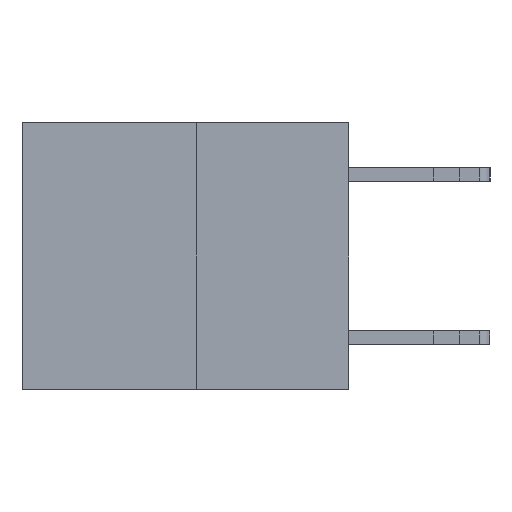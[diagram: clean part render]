
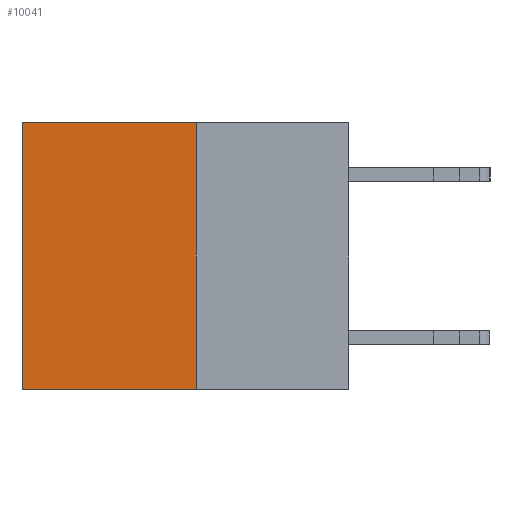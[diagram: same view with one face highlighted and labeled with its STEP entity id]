
A CAD part, left-side view. The second image highlights one B-rep face of the part: STEP entity #10041.
In plain terms, the highlighted planar face has unit normal (-1, 0, 0).
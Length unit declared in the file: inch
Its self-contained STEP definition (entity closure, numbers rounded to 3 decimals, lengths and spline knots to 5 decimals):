
#170 = PLANE ( 'NONE',  #9538 ) ;
#248 = CARTESIAN_POINT ( 'NONE',  ( 0.3165, 0.28, -0.49 ) ) ;
#251 = DIRECTION ( 'NONE',  ( 0., 1., 0. ) ) ;
#1342 = ORIENTED_EDGE ( 'NONE', *, *, #8100, .F. ) ;
#1426 = EDGE_CURVE ( 'NONE', #12046, #2848, #7348, .T. ) ;
#1873 = EDGE_LOOP ( 'NONE', ( #5489, #9481, #1342, #3437 ) ) ;
#2848 = VERTEX_POINT ( 'NONE', #3952 ) ;
#2997 = EDGE_CURVE ( 'NONE', #3380, #7365, #10360, .T. ) ;
#3380 = VERTEX_POINT ( 'NONE', #11520 ) ;
#3437 = ORIENTED_EDGE ( 'NONE', *, *, #1426, .T. ) ;
#3952 = CARTESIAN_POINT ( 'NONE',  ( 0.3165, 0.6, 0. ) ) ;
#4978 = LINE ( 'NONE', #10713, #12316 ) ;
#5038 = VECTOR ( 'NONE', #5863, 39.37008 ) ;
#5358 = CARTESIAN_POINT ( 'NONE',  ( 0.3165, 0.28, 0. ) ) ;
#5463 = VECTOR ( 'NONE', #251, 39.37008 ) ;
#5489 = ORIENTED_EDGE ( 'NONE', *, *, #10489, .T. ) ;
#5657 = DIRECTION ( 'NONE',  ( 0., 0., -1. ) ) ;
#5863 = DIRECTION ( 'NONE',  ( 0., 1., 0. ) ) ;
#6098 = CARTESIAN_POINT ( 'NONE',  ( 0.3165, 0.28, -0.49 ) ) ;
#6902 = DIRECTION ( 'NONE',  ( 1., 0., 0. ) ) ;
#7070 = VECTOR ( 'NONE', #5657, 39.37008 ) ;
#7348 = LINE ( 'NONE', #10740, #5038 ) ;
#7365 = VERTEX_POINT ( 'NONE', #9701 ) ;
#7507 = CARTESIAN_POINT ( 'NONE',  ( 0.3165, 0.28, -0.49 ) ) ;
#7882 = DIRECTION ( 'NONE',  ( 0., 0., -1. ) ) ;
#7975 = LINE ( 'NONE', #7507, #7070 ) ;
#8100 = EDGE_CURVE ( 'NONE', #12046, #3380, #7975, .T. ) ;
#9481 = ORIENTED_EDGE ( 'NONE', *, *, #2997, .F. ) ;
#9538 = AXIS2_PLACEMENT_3D ( 'NONE', #248, #6902, #7882 ) ;
#9701 = CARTESIAN_POINT ( 'NONE',  ( 0.3165, 0.6, -0.49 ) ) ;
#9763 = DIRECTION ( 'NONE',  ( 0., 0., -1. ) ) ;
#10041 = ADVANCED_FACE ( 'NONE', ( #10659 ), #170, .F. ) ;
#10360 = LINE ( 'NONE', #6098, #5463 ) ;
#10489 = EDGE_CURVE ( 'NONE', #2848, #7365, #4978, .T. ) ;
#10659 = FACE_OUTER_BOUND ( 'NONE', #1873, .T. ) ;
#10713 = CARTESIAN_POINT ( 'NONE',  ( 0.3165, 0.6, -0.49 ) ) ;
#10740 = CARTESIAN_POINT ( 'NONE',  ( 0.3165, 0.28, 0. ) ) ;
#11520 = CARTESIAN_POINT ( 'NONE',  ( 0.3165, 0.28, -0.49 ) ) ;
#12046 = VERTEX_POINT ( 'NONE', #5358 ) ;
#12316 = VECTOR ( 'NONE', #9763, 39.37008 ) ;
